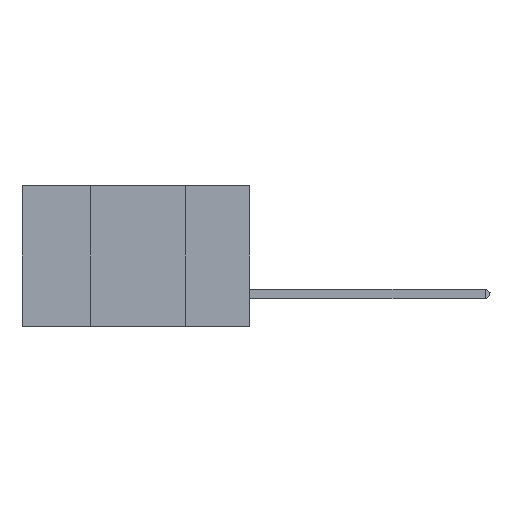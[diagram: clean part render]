
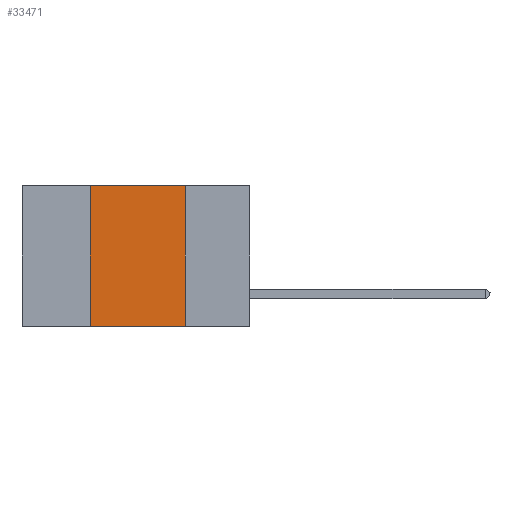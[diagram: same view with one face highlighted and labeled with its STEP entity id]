
A CAD part, left-side view. The second image highlights one B-rep face of the part: STEP entity #33471.
In plain terms, the highlighted planar face has unit normal (-1, 0, 0).
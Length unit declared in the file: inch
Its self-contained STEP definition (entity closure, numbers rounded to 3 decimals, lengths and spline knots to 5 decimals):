
#1385 = PLANE ( 'NONE',  #33108 ) ;
#1699 = EDGE_LOOP ( 'NONE', ( #30188, #16655, #6383, #16908 ) ) ;
#4069 = CARTESIAN_POINT ( 'NONE',  ( 0., 0.42, 0. ) ) ;
#4643 = LINE ( 'NONE', #16644, #37654 ) ;
#6264 = DIRECTION ( 'NONE',  ( 0., -1., 0. ) ) ;
#6383 = ORIENTED_EDGE ( 'NONE', *, *, #34118, .F. ) ;
#7374 = EDGE_CURVE ( 'NONE', #21854, #9686, #26948, .T. ) ;
#9686 = VERTEX_POINT ( 'NONE', #38520 ) ;
#10326 = DIRECTION ( 'NONE',  ( 0., 0., -1. ) ) ;
#10912 = DIRECTION ( 'NONE',  ( 0., -1., 0. ) ) ;
#13431 = CARTESIAN_POINT ( 'NONE',  ( 0., 0.6, 0. ) ) ;
#14112 = EDGE_CURVE ( 'NONE', #31073, #21854, #18975, .T. ) ;
#15802 = DIRECTION ( 'NONE',  ( 0., 0., -1. ) ) ;
#16644 = CARTESIAN_POINT ( 'NONE',  ( 0., 0.42, 0. ) ) ;
#16655 = ORIENTED_EDGE ( 'NONE', *, *, #14112, .F. ) ;
#16908 = ORIENTED_EDGE ( 'NONE', *, *, #21262, .T. ) ;
#17620 = VECTOR ( 'NONE', #15802, 39.37008 ) ;
#18961 = VECTOR ( 'NONE', #10912, 39.37008 ) ;
#18975 = LINE ( 'NONE', #30226, #28810 ) ;
#19839 = CARTESIAN_POINT ( 'NONE',  ( 0., 0.6, -0.37 ) ) ;
#21262 = EDGE_CURVE ( 'NONE', #27063, #9686, #34850, .T. ) ;
#21854 = VERTEX_POINT ( 'NONE', #35084 ) ;
#25044 = CARTESIAN_POINT ( 'NONE',  ( 0., 0.17, 0. ) ) ;
#25636 = FACE_OUTER_BOUND ( 'NONE', #1699, .T. ) ;
#26948 = LINE ( 'NONE', #25044, #17620 ) ;
#27063 = VERTEX_POINT ( 'NONE', #30037 ) ;
#28154 = DIRECTION ( 'NONE',  ( 1., 0., 0. ) ) ;
#28631 = DIRECTION ( 'NONE',  ( 0., 0., 1. ) ) ;
#28810 = VECTOR ( 'NONE', #6264, 39.37008 ) ;
#30037 = CARTESIAN_POINT ( 'NONE',  ( 0., 0.42, -0.37 ) ) ;
#30188 = ORIENTED_EDGE ( 'NONE', *, *, #7374, .F. ) ;
#30226 = CARTESIAN_POINT ( 'NONE',  ( 0., 0.6, 0. ) ) ;
#31073 = VERTEX_POINT ( 'NONE', #4069 ) ;
#33108 = AXIS2_PLACEMENT_3D ( 'NONE', #13431, #28154, #10326 ) ;
#33471 = ADVANCED_FACE ( 'NONE', ( #25636 ), #1385, .F. ) ;
#34118 = EDGE_CURVE ( 'NONE', #27063, #31073, #4643, .T. ) ;
#34850 = LINE ( 'NONE', #19839, #18961 ) ;
#35084 = CARTESIAN_POINT ( 'NONE',  ( 0., 0.17, 0. ) ) ;
#37654 = VECTOR ( 'NONE', #28631, 39.37008 ) ;
#38520 = CARTESIAN_POINT ( 'NONE',  ( 0., 0.17, -0.37 ) ) ;
